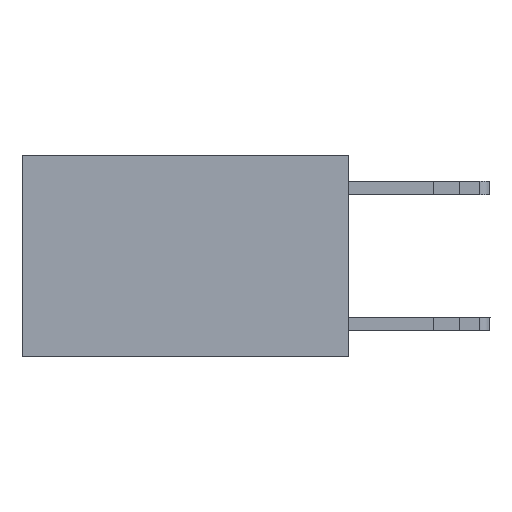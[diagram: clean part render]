
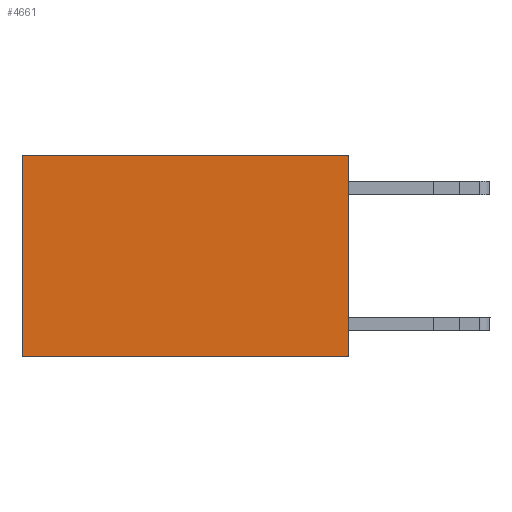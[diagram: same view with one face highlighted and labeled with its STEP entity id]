
A CAD part, left-side view. The second image highlights one B-rep face of the part: STEP entity #4661.
In plain terms, the highlighted planar face has unit normal (-1, 0, 0).
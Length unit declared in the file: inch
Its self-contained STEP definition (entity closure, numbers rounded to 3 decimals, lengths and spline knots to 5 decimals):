
#56 = VERTEX_POINT ( 'NONE', #6084 ) ;
#256 = EDGE_CURVE ( 'NONE', #7115, #1856, #3111, .T. ) ;
#273 = ORIENTED_EDGE ( 'NONE', *, *, #5206, .T. ) ;
#392 = EDGE_CURVE ( 'NONE', #3794, #56, #7554, .T. ) ;
#648 = PLANE ( 'NONE',  #1153 ) ;
#1153 = AXIS2_PLACEMENT_3D ( 'NONE', #7118, #8171, #1898 ) ;
#1815 = CARTESIAN_POINT ( 'NONE',  ( 0.2625, 0., 0. ) ) ;
#1856 = VERTEX_POINT ( 'NONE', #7362 ) ;
#1898 = DIRECTION ( 'NONE',  ( 0., 0., -1. ) ) ;
#2797 = VECTOR ( 'NONE', #5194, 39.37008 ) ;
#3111 = LINE ( 'NONE', #6497, #2797 ) ;
#3717 = ORIENTED_EDGE ( 'NONE', *, *, #392, .T. ) ;
#3794 = VERTEX_POINT ( 'NONE', #1815 ) ;
#3957 = CARTESIAN_POINT ( 'NONE',  ( 0.2625, 0., -0.37 ) ) ;
#4355 = EDGE_LOOP ( 'NONE', ( #273, #4445, #5063, #3717 ) ) ;
#4445 = ORIENTED_EDGE ( 'NONE', *, *, #256, .F. ) ;
#4604 = CARTESIAN_POINT ( 'NONE',  ( 0.2625, 0., 0. ) ) ;
#4661 = ADVANCED_FACE ( 'NONE', ( #5745 ), #648, .F. ) ;
#4781 = VECTOR ( 'NONE', #9583, 39.37008 ) ;
#5063 = ORIENTED_EDGE ( 'NONE', *, *, #9179, .F. ) ;
#5194 = DIRECTION ( 'NONE',  ( 0., 1., 0. ) ) ;
#5206 = EDGE_CURVE ( 'NONE', #56, #1856, #10814, .T. ) ;
#5731 = VECTOR ( 'NONE', #12893, 39.37008 ) ;
#5745 = FACE_OUTER_BOUND ( 'NONE', #4355, .T. ) ;
#6084 = CARTESIAN_POINT ( 'NONE',  ( 0.2625, 0.6, 0. ) ) ;
#6137 = DIRECTION ( 'NONE',  ( 0., 0., -1. ) ) ;
#6319 = VECTOR ( 'NONE', #6137, 39.37008 ) ;
#6497 = CARTESIAN_POINT ( 'NONE',  ( 0.2625, 0., -0.37 ) ) ;
#7115 = VERTEX_POINT ( 'NONE', #3957 ) ;
#7118 = CARTESIAN_POINT ( 'NONE',  ( 0.2625, 0., 0. ) ) ;
#7362 = CARTESIAN_POINT ( 'NONE',  ( 0.2625, 0.6, -0.37 ) ) ;
#7554 = LINE ( 'NONE', #4604, #4781 ) ;
#8171 = DIRECTION ( 'NONE',  ( 1., 0., 0. ) ) ;
#9179 = EDGE_CURVE ( 'NONE', #3794, #7115, #11987, .T. ) ;
#9583 = DIRECTION ( 'NONE',  ( 0., 1., 0. ) ) ;
#10814 = LINE ( 'NONE', #10897, #5731 ) ;
#10897 = CARTESIAN_POINT ( 'NONE',  ( 0.2625, 0.6, 0. ) ) ;
#11987 = LINE ( 'NONE', #13176, #6319 ) ;
#12893 = DIRECTION ( 'NONE',  ( 0., 0., -1. ) ) ;
#13176 = CARTESIAN_POINT ( 'NONE',  ( 0.2625, 0., 0. ) ) ;
